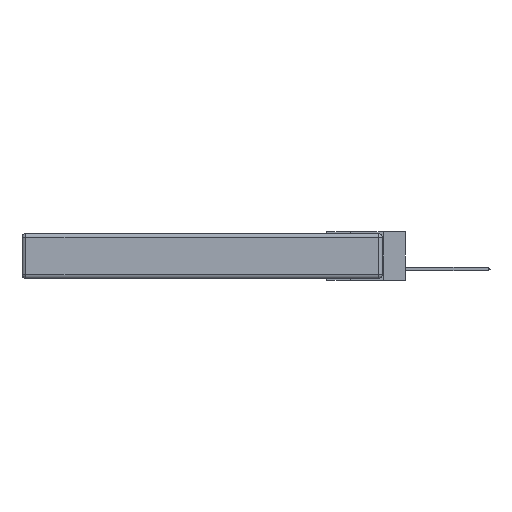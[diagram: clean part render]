
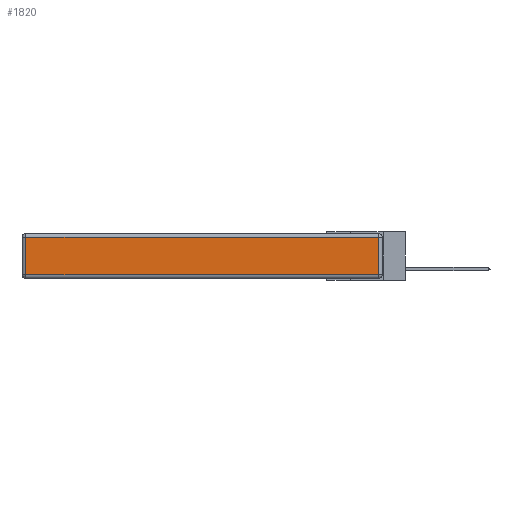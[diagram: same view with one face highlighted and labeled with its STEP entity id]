
A CAD part, left-side view. The second image highlights one B-rep face of the part: STEP entity #1820.
In plain terms, the highlighted planar face has unit normal (-1, 0, 0).
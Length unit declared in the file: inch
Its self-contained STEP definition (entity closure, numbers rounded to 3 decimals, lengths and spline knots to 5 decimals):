
#28 = AXIS2_PLACEMENT_3D ( 'NONE', #906, #10570, #5195 ) ;
#906 = CARTESIAN_POINT ( 'NONE',  ( 0., 0., -0.343 ) ) ;
#1820 = ADVANCED_FACE ( 'NONE', ( #6664 ), #14532, .T. ) ;
#1950 = CARTESIAN_POINT ( 'NONE',  ( 0., 2.75, -0.03 ) ) ;
#1960 = ORIENTED_EDGE ( 'NONE', *, *, #17371, .T. ) ;
#1999 = DIRECTION ( 'NONE',  ( 0., -1., 0. ) ) ;
#2182 = LINE ( 'NONE', #16705, #10840 ) ;
#3074 = CARTESIAN_POINT ( 'NONE',  ( 0., 2.72, -0.313 ) ) ;
#5071 = VECTOR ( 'NONE', #7382, 39.37008 ) ;
#5195 = DIRECTION ( 'NONE',  ( 0., 0., 1. ) ) ;
#5487 = LINE ( 'NONE', #7565, #5071 ) ;
#5885 = EDGE_LOOP ( 'NONE', ( #14400, #9487, #1960, #16141 ) ) ;
#6664 = FACE_OUTER_BOUND ( 'NONE', #5885, .T. ) ;
#7038 = EDGE_CURVE ( 'NONE', #13826, #9539, #5487, .T. ) ;
#7211 = LINE ( 'NONE', #17197, #8078 ) ;
#7382 = DIRECTION ( 'NONE',  ( 0., 0., -1. ) ) ;
#7414 = VECTOR ( 'NONE', #11348, 39.37008 ) ;
#7565 = CARTESIAN_POINT ( 'NONE',  ( 0., 2.72, -0.343 ) ) ;
#8078 = VECTOR ( 'NONE', #1999, 39.37008 ) ;
#9487 = ORIENTED_EDGE ( 'NONE', *, *, #10141, .T. ) ;
#9539 = VERTEX_POINT ( 'NONE', #3074 ) ;
#9610 = CARTESIAN_POINT ( 'NONE',  ( 0., 0.03, -0.03 ) ) ;
#9786 = DIRECTION ( 'NONE',  ( 0., 0., 1. ) ) ;
#10141 = EDGE_CURVE ( 'NONE', #10707, #15784, #2182, .T. ) ;
#10570 = DIRECTION ( 'NONE',  ( -1., 0., 0. ) ) ;
#10707 = VERTEX_POINT ( 'NONE', #15858 ) ;
#10840 = VECTOR ( 'NONE', #9786, 39.37008 ) ;
#11348 = DIRECTION ( 'NONE',  ( 0., 1., 0. ) ) ;
#11557 = EDGE_CURVE ( 'NONE', #9539, #10707, #7211, .T. ) ;
#11642 = LINE ( 'NONE', #1950, #7414 ) ;
#13826 = VERTEX_POINT ( 'NONE', #17001 ) ;
#14400 = ORIENTED_EDGE ( 'NONE', *, *, #11557, .T. ) ;
#14532 = PLANE ( 'NONE',  #28 ) ;
#15784 = VERTEX_POINT ( 'NONE', #9610 ) ;
#15858 = CARTESIAN_POINT ( 'NONE',  ( 0., 0.03, -0.313 ) ) ;
#16141 = ORIENTED_EDGE ( 'NONE', *, *, #7038, .T. ) ;
#16705 = CARTESIAN_POINT ( 'NONE',  ( 0., 0.03, -0.343 ) ) ;
#17001 = CARTESIAN_POINT ( 'NONE',  ( 0., 2.72, -0.03 ) ) ;
#17197 = CARTESIAN_POINT ( 'NONE',  ( 0., 0., -0.313 ) ) ;
#17371 = EDGE_CURVE ( 'NONE', #15784, #13826, #11642, .T. ) ;
